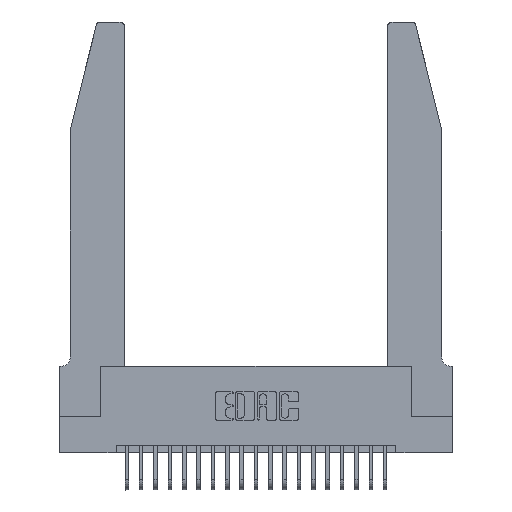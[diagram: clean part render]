
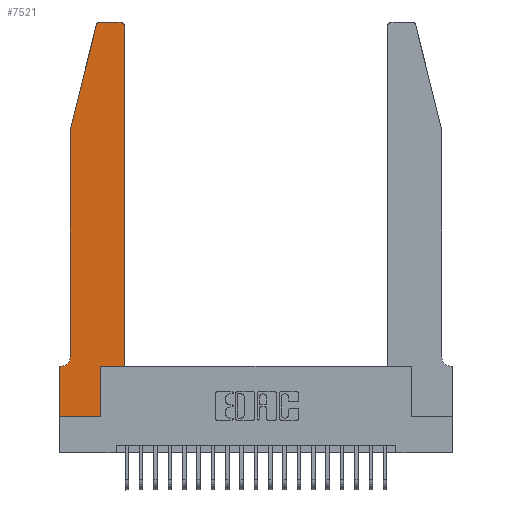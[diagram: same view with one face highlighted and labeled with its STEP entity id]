
A CAD part, top view. The second image highlights one B-rep face of the part: STEP entity #7521.
In plain terms, the highlighted planar face has unit normal (0, 0, 1).
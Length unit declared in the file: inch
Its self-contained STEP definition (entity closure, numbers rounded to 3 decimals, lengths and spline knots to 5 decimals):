
#283 = DIRECTION ( 'NONE',  ( -1., 0., 0. ) ) ;
#392 = EDGE_CURVE ( 'NONE', #3159, #1498, #19643, .T. ) ;
#953 = CARTESIAN_POINT ( 'NONE',  ( 0.2865, 0.35, 0.37 ) ) ;
#1280 = EDGE_CURVE ( 'NONE', #21896, #12960, #2993, .T. ) ;
#1498 = VERTEX_POINT ( 'NONE', #5479 ) ;
#1501 = AXIS2_PLACEMENT_3D ( 'NONE', #15749, #3718, #14021 ) ;
#1530 = ORIENTED_EDGE ( 'NONE', *, *, #11064, .T. ) ;
#1700 = CARTESIAN_POINT ( 'NONE',  ( 0.0755, 2., 0.37 ) ) ;
#1774 = DIRECTION ( 'NONE',  ( 1., 0., 0. ) ) ;
#1880 = ORIENTED_EDGE ( 'NONE', *, *, #11832, .T. ) ;
#1928 = EDGE_CURVE ( 'NONE', #10074, #10865, #12350, .T. ) ;
#1999 = DIRECTION ( 'NONE',  ( 0., -1., 0. ) ) ;
#2507 = VERTEX_POINT ( 'NONE', #18857 ) ;
#2552 = VECTOR ( 'NONE', #1999, 39.37008 ) ;
#2921 = VECTOR ( 'NONE', #283, 39.37008 ) ;
#2993 = LINE ( 'NONE', #1700, #7700 ) ;
#3159 = VERTEX_POINT ( 'NONE', #7454 ) ;
#3313 = DIRECTION ( 'NONE',  ( -1., 0., 0. ) ) ;
#3476 = LINE ( 'NONE', #20934, #2921 ) ;
#3488 = EDGE_LOOP ( 'NONE', ( #1880, #19422, #17679, #14873, #20317, #4376, #15742, #10731, #9900, #19778, #1530, #4130 ) ) ;
#3490 = VECTOR ( 'NONE', #16802, 39.37008 ) ;
#3675 = EDGE_CURVE ( 'NONE', #8611, #13316, #14395, .T. ) ;
#3718 = DIRECTION ( 'NONE',  ( 0., 0., -1. ) ) ;
#3995 = CARTESIAN_POINT ( 'NONE',  ( 0., 0.35, 0.37 ) ) ;
#4053 = LINE ( 'NONE', #15125, #3490 ) ;
#4130 = ORIENTED_EDGE ( 'NONE', *, *, #3675, .T. ) ;
#4376 = ORIENTED_EDGE ( 'NONE', *, *, #8111, .T. ) ;
#4744 = CARTESIAN_POINT ( 'NONE',  ( 0.4205, 2.75, 0.37 ) ) ;
#5417 = LINE ( 'NONE', #8307, #14013 ) ;
#5479 = CARTESIAN_POINT ( 'NONE',  ( 0.0055, 0.35, 0.37 ) ) ;
#5655 = DIRECTION ( 'NONE',  ( 0., 0., 1. ) ) ;
#6037 = CARTESIAN_POINT ( 'NONE',  ( 0.0755, 2., 0.37 ) ) ;
#6459 = FACE_OUTER_BOUND ( 'NONE', #3488, .T. ) ;
#7454 = CARTESIAN_POINT ( 'NONE',  ( 0.0755, 0.42, 0.37 ) ) ;
#7521 = ADVANCED_FACE ( 'NONE', ( #6459 ), #22200, .T. ) ;
#7700 = VECTOR ( 'NONE', #8654, 39.37008 ) ;
#7727 = CIRCLE ( 'NONE', #15406, 0.03 ) ;
#8111 = EDGE_CURVE ( 'NONE', #1498, #10074, #3476, .T. ) ;
#8112 = DIRECTION ( 'NONE',  ( 0., 1., 0. ) ) ;
#8307 = CARTESIAN_POINT ( 'NONE',  ( 0., 0., 0.37 ) ) ;
#8533 = CARTESIAN_POINT ( 'NONE',  ( 0.0755, 2., 0.37 ) ) ;
#8611 = VERTEX_POINT ( 'NONE', #18915 ) ;
#8654 = DIRECTION ( 'NONE',  ( -0.239, -0.971, 0. ) ) ;
#9774 = DIRECTION ( 'NONE',  ( 0., 0., 1. ) ) ;
#9900 = ORIENTED_EDGE ( 'NONE', *, *, #16446, .T. ) ;
#10074 = VERTEX_POINT ( 'NONE', #3995 ) ;
#10279 = CARTESIAN_POINT ( 'NONE',  ( 0.284, 2.75, 0.37 ) ) ;
#10359 = EDGE_CURVE ( 'NONE', #12960, #3159, #19464, .T. ) ;
#10731 = ORIENTED_EDGE ( 'NONE', *, *, #19964, .T. ) ;
#10865 = VERTEX_POINT ( 'NONE', #21142 ) ;
#11064 = EDGE_CURVE ( 'NONE', #15936, #8611, #22067, .T. ) ;
#11624 = VERTEX_POINT ( 'NONE', #953 ) ;
#11698 = CARTESIAN_POINT ( 'NONE',  ( 0.4505, 0.35, 0.37 ) ) ;
#11832 = EDGE_CURVE ( 'NONE', #13316, #18341, #16254, .T. ) ;
#11983 = CARTESIAN_POINT ( 'NONE',  ( 0.2605, 2.75, 0.37 ) ) ;
#12208 = DIRECTION ( 'NONE',  ( 0., 0., 1. ) ) ;
#12350 = LINE ( 'NONE', #19100, #2552 ) ;
#12792 = EDGE_CURVE ( 'NONE', #18341, #21896, #7727, .T. ) ;
#12960 = VERTEX_POINT ( 'NONE', #8533 ) ;
#13316 = VERTEX_POINT ( 'NONE', #4744 ) ;
#14013 = VECTOR ( 'NONE', #21842, 39.37008 ) ;
#14021 = DIRECTION ( 'NONE',  ( -1., 0., 0. ) ) ;
#14395 = CIRCLE ( 'NONE', #16145, 0.03 ) ;
#14864 = CARTESIAN_POINT ( 'NONE',  ( 0.2865, 0.35, 0.37 ) ) ;
#14873 = ORIENTED_EDGE ( 'NONE', *, *, #10359, .T. ) ;
#14900 = CARTESIAN_POINT ( 'NONE',  ( 0.4505, 0.35, 0.37 ) ) ;
#15125 = CARTESIAN_POINT ( 'NONE',  ( 0.4505, 0.35, 0.37 ) ) ;
#15406 = AXIS2_PLACEMENT_3D ( 'NONE', #19876, #9774, #21584 ) ;
#15742 = ORIENTED_EDGE ( 'NONE', *, *, #1928, .T. ) ;
#15749 = CARTESIAN_POINT ( 'NONE',  ( 0.0055, 0.42, 0.37 ) ) ;
#15879 = CARTESIAN_POINT ( 'NONE',  ( 0.4205, 2.72, 0.37 ) ) ;
#15936 = VERTEX_POINT ( 'NONE', #11698 ) ;
#16145 = AXIS2_PLACEMENT_3D ( 'NONE', #15879, #5655, #17557 ) ;
#16254 = LINE ( 'NONE', #11983, #20175 ) ;
#16446 = EDGE_CURVE ( 'NONE', #2507, #11624, #16535, .T. ) ;
#16535 = LINE ( 'NONE', #14864, #19934 ) ;
#16802 = DIRECTION ( 'NONE',  ( 1., 0., 0. ) ) ;
#17557 = DIRECTION ( 'NONE',  ( 1., 0., 0. ) ) ;
#17590 = VECTOR ( 'NONE', #8112, 39.37008 ) ;
#17679 = ORIENTED_EDGE ( 'NONE', *, *, #1280, .T. ) ;
#17922 = DIRECTION ( 'NONE',  ( 0., -1., 0. ) ) ;
#18225 = DIRECTION ( 'NONE',  ( 0., 1., 0. ) ) ;
#18307 = AXIS2_PLACEMENT_3D ( 'NONE', #20573, #12208, #1774 ) ;
#18341 = VERTEX_POINT ( 'NONE', #10279 ) ;
#18857 = CARTESIAN_POINT ( 'NONE',  ( 0.2865, 0., 0.37 ) ) ;
#18915 = CARTESIAN_POINT ( 'NONE',  ( 0.4505, 2.72, 0.37 ) ) ;
#18939 = VECTOR ( 'NONE', #17922, 39.37008 ) ;
#19100 = CARTESIAN_POINT ( 'NONE',  ( 0., 0., 0.37 ) ) ;
#19361 = EDGE_CURVE ( 'NONE', #11624, #15936, #4053, .T. ) ;
#19422 = ORIENTED_EDGE ( 'NONE', *, *, #12792, .T. ) ;
#19464 = LINE ( 'NONE', #6037, #18939 ) ;
#19476 = CARTESIAN_POINT ( 'NONE',  ( 0.25487, 2.72718, 0.37 ) ) ;
#19643 = CIRCLE ( 'NONE', #1501, 0.07 ) ;
#19778 = ORIENTED_EDGE ( 'NONE', *, *, #19361, .T. ) ;
#19876 = CARTESIAN_POINT ( 'NONE',  ( 0.284, 2.72, 0.37 ) ) ;
#19934 = VECTOR ( 'NONE', #18225, 39.37008 ) ;
#19964 = EDGE_CURVE ( 'NONE', #10865, #2507, #5417, .T. ) ;
#20175 = VECTOR ( 'NONE', #3313, 39.37008 ) ;
#20317 = ORIENTED_EDGE ( 'NONE', *, *, #392, .T. ) ;
#20573 = CARTESIAN_POINT ( 'NONE',  ( 0., 0.35, 0.37 ) ) ;
#20934 = CARTESIAN_POINT ( 'NONE',  ( 0.0755, 0.35, 0.37 ) ) ;
#21142 = CARTESIAN_POINT ( 'NONE',  ( 0., 0., 0.37 ) ) ;
#21584 = DIRECTION ( 'NONE',  ( 1., 0., 0. ) ) ;
#21842 = DIRECTION ( 'NONE',  ( 1., 0., 0. ) ) ;
#21896 = VERTEX_POINT ( 'NONE', #19476 ) ;
#22067 = LINE ( 'NONE', #14900, #17590 ) ;
#22200 = PLANE ( 'NONE',  #18307 ) ;
